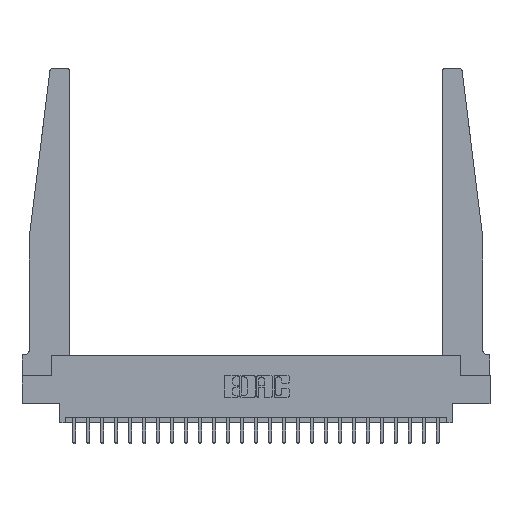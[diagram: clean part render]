
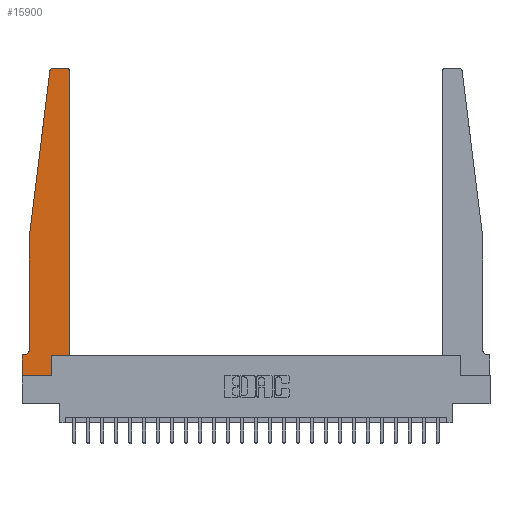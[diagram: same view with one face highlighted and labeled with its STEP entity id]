
A CAD part, top view. The second image highlights one B-rep face of the part: STEP entity #15900.
In plain terms, the highlighted planar face has unit normal (0, 0, 1).
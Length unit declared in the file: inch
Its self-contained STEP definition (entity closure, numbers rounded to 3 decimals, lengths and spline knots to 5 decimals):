
#235 = DIRECTION ( 'NONE',  ( 0., 0., -1. ) ) ;
#636 = DIRECTION ( 'NONE',  ( 0., 0., 1. ) ) ;
#712 = DIRECTION ( 'NONE',  ( -1., 0., 0. ) ) ;
#1125 = EDGE_CURVE ( 'NONE', #11993, #11760, #8908, .T. ) ;
#1441 = CARTESIAN_POINT ( 'NONE',  ( 0., 0., 0.37 ) ) ;
#2278 = CARTESIAN_POINT ( 'NONE',  ( 0.2605, 0.18, 0.37 ) ) ;
#2827 = CARTESIAN_POINT ( 'NONE',  ( 0.27653, 2.75, 0.37 ) ) ;
#3395 = CARTESIAN_POINT ( 'NONE',  ( 0.25, 2.75, 0.37 ) ) ;
#3466 = DIRECTION ( 'NONE',  ( -1., 0., 0. ) ) ;
#3523 = LINE ( 'NONE', #1441, #18230 ) ;
#3990 = CARTESIAN_POINT ( 'NONE',  ( 0.425, 0.18, 0.37 ) ) ;
#4384 = LINE ( 'NONE', #20730, #14034 ) ;
#4577 = VERTEX_POINT ( 'NONE', #5145 ) ;
#5145 = CARTESIAN_POINT ( 'NONE',  ( 0.24675, 2.72367, 0.37 ) ) ;
#5497 = VERTEX_POINT ( 'NONE', #19209 ) ;
#5551 = CARTESIAN_POINT ( 'NONE',  ( 0.065, 0.2375, 0.37 ) ) ;
#5699 = EDGE_CURVE ( 'NONE', #8540, #6221, #24398, .T. ) ;
#6221 = VERTEX_POINT ( 'NONE', #3990 ) ;
#6239 = CARTESIAN_POINT ( 'NONE',  ( 0.2605, 0., 0.37 ) ) ;
#7141 = EDGE_CURVE ( 'NONE', #9320, #12392, #3523, .T. ) ;
#7371 = DIRECTION ( 'NONE',  ( -0.122, -0.992, 0. ) ) ;
#7680 = CARTESIAN_POINT ( 'NONE',  ( 0.065, 1.25, 0.37 ) ) ;
#7788 = DIRECTION ( 'NONE',  ( 0., 0., 1. ) ) ;
#7808 = EDGE_CURVE ( 'NONE', #4577, #15615, #4384, .T. ) ;
#8377 = LINE ( 'NONE', #21371, #17964 ) ;
#8540 = VERTEX_POINT ( 'NONE', #24537 ) ;
#8908 = LINE ( 'NONE', #3395, #13437 ) ;
#9320 = VERTEX_POINT ( 'NONE', #13478 ) ;
#9577 = CARTESIAN_POINT ( 'NONE',  ( 0.395, 2.75, 0.37 ) ) ;
#9990 = DIRECTION ( 'NONE',  ( 1., 0., 0. ) ) ;
#10192 = CARTESIAN_POINT ( 'NONE',  ( 0.425, 0.18, 0.37 ) ) ;
#10395 = DIRECTION ( 'NONE',  ( 0., 0., 1. ) ) ;
#10892 = EDGE_CURVE ( 'NONE', #10963, #8540, #19059, .T. ) ;
#10963 = VERTEX_POINT ( 'NONE', #6239 ) ;
#11514 = VECTOR ( 'NONE', #712, 39.37008 ) ;
#11760 = VERTEX_POINT ( 'NONE', #2827 ) ;
#11871 = CARTESIAN_POINT ( 'NONE',  ( 0.015, 0.2375, 0.37 ) ) ;
#11993 = VERTEX_POINT ( 'NONE', #9577 ) ;
#12270 = CARTESIAN_POINT ( 'NONE',  ( 0.395, 2.72, 0.37 ) ) ;
#12392 = VERTEX_POINT ( 'NONE', #16525 ) ;
#13134 = VERTEX_POINT ( 'NONE', #5551 ) ;
#13417 = VECTOR ( 'NONE', #17672, 39.37008 ) ;
#13437 = VECTOR ( 'NONE', #3466, 39.37008 ) ;
#13478 = CARTESIAN_POINT ( 'NONE',  ( 0., 0.1875, 0.37 ) ) ;
#13790 = DIRECTION ( 'NONE',  ( -1., 0., 0. ) ) ;
#13809 = AXIS2_PLACEMENT_3D ( 'NONE', #12270, #636, #14163 ) ;
#14034 = VECTOR ( 'NONE', #7371, 39.37008 ) ;
#14163 = DIRECTION ( 'NONE',  ( 1., 0., 0. ) ) ;
#14381 = FACE_OUTER_BOUND ( 'NONE', #15204, .T. ) ;
#15075 = EDGE_CURVE ( 'NONE', #11760, #4577, #17723, .T. ) ;
#15204 = EDGE_LOOP ( 'NONE', ( #22504, #22596, #22715, #22864, #22938, #23156, #23197, #23414, #23441, #23737, #24013, #24129 ) ) ;
#15549 = EDGE_CURVE ( 'NONE', #6221, #5497, #17109, .T. ) ;
#15615 = VERTEX_POINT ( 'NONE', #7680 ) ;
#15698 = CARTESIAN_POINT ( 'NONE',  ( 0.065, 1.25, 0.37 ) ) ;
#15900 = ADVANCED_FACE ( 'NONE', ( #14381 ), #21743, .T. ) ;
#15959 = DIRECTION ( 'NONE',  ( 1., 0., 0. ) ) ;
#16165 = CIRCLE ( 'NONE', #17100, 0.05 ) ;
#16352 = EDGE_CURVE ( 'NONE', #13134, #22639, #16165, .T. ) ;
#16525 = CARTESIAN_POINT ( 'NONE',  ( 0., 0., 0.37 ) ) ;
#16611 = CIRCLE ( 'NONE', #13809, 0.03 ) ;
#16708 = LINE ( 'NONE', #15698, #21697 ) ;
#17048 = EDGE_CURVE ( 'NONE', #12392, #10963, #8377, .T. ) ;
#17100 = AXIS2_PLACEMENT_3D ( 'NONE', #11871, #235, #13790 ) ;
#17109 = LINE ( 'NONE', #20861, #21506 ) ;
#17138 = VECTOR ( 'NONE', #15959, 39.37008 ) ;
#17567 = AXIS2_PLACEMENT_3D ( 'NONE', #17967, #10395, #23605 ) ;
#17672 = DIRECTION ( 'NONE',  ( 0., 1., 0. ) ) ;
#17691 = DIRECTION ( 'NONE',  ( 0., -1., 0. ) ) ;
#17723 = CIRCLE ( 'NONE', #20212, 0.03 ) ;
#17964 = VECTOR ( 'NONE', #9990, 39.37008 ) ;
#17967 = CARTESIAN_POINT ( 'NONE',  ( 0., 0.1875, 0.37 ) ) ;
#18230 = VECTOR ( 'NONE', #20599, 39.37008 ) ;
#19059 = LINE ( 'NONE', #2278, #13417 ) ;
#19209 = CARTESIAN_POINT ( 'NONE',  ( 0.425, 2.72, 0.37 ) ) ;
#19267 = CARTESIAN_POINT ( 'NONE',  ( 0.27653, 2.72, 0.37 ) ) ;
#19539 = EDGE_CURVE ( 'NONE', #15615, #13134, #16708, .T. ) ;
#20212 = AXIS2_PLACEMENT_3D ( 'NONE', #19267, #7788, #21137 ) ;
#20501 = CARTESIAN_POINT ( 'NONE',  ( 0.015, 0.1875, 0.37 ) ) ;
#20599 = DIRECTION ( 'NONE',  ( 0., -1., 0. ) ) ;
#20730 = CARTESIAN_POINT ( 'NONE',  ( 0.065, 1.25, 0.37 ) ) ;
#20861 = CARTESIAN_POINT ( 'NONE',  ( 0.425, 0.18, 0.37 ) ) ;
#21137 = DIRECTION ( 'NONE',  ( 1., 0., 0. ) ) ;
#21371 = CARTESIAN_POINT ( 'NONE',  ( 0., 0., 0.37 ) ) ;
#21398 = EDGE_CURVE ( 'NONE', #5497, #11993, #16611, .T. ) ;
#21506 = VECTOR ( 'NONE', #22732, 39.37008 ) ;
#21697 = VECTOR ( 'NONE', #17691, 39.37008 ) ;
#21743 = PLANE ( 'NONE',  #17567 ) ;
#21859 = EDGE_CURVE ( 'NONE', #22639, #9320, #22166, .T. ) ;
#22166 = LINE ( 'NONE', #23635, #11514 ) ;
#22504 = ORIENTED_EDGE ( 'NONE', *, *, #1125, .T. ) ;
#22596 = ORIENTED_EDGE ( 'NONE', *, *, #15075, .T. ) ;
#22639 = VERTEX_POINT ( 'NONE', #20501 ) ;
#22715 = ORIENTED_EDGE ( 'NONE', *, *, #7808, .T. ) ;
#22732 = DIRECTION ( 'NONE',  ( 0., 1., 0. ) ) ;
#22864 = ORIENTED_EDGE ( 'NONE', *, *, #19539, .T. ) ;
#22938 = ORIENTED_EDGE ( 'NONE', *, *, #16352, .T. ) ;
#23156 = ORIENTED_EDGE ( 'NONE', *, *, #21859, .T. ) ;
#23197 = ORIENTED_EDGE ( 'NONE', *, *, #7141, .T. ) ;
#23414 = ORIENTED_EDGE ( 'NONE', *, *, #17048, .T. ) ;
#23441 = ORIENTED_EDGE ( 'NONE', *, *, #10892, .T. ) ;
#23605 = DIRECTION ( 'NONE',  ( 1., 0., 0. ) ) ;
#23635 = CARTESIAN_POINT ( 'NONE',  ( 0.065, 0.1875, 0.37 ) ) ;
#23737 = ORIENTED_EDGE ( 'NONE', *, *, #5699, .T. ) ;
#24013 = ORIENTED_EDGE ( 'NONE', *, *, #15549, .T. ) ;
#24129 = ORIENTED_EDGE ( 'NONE', *, *, #21398, .T. ) ;
#24398 = LINE ( 'NONE', #10192, #17138 ) ;
#24537 = CARTESIAN_POINT ( 'NONE',  ( 0.2605, 0.18, 0.37 ) ) ;
